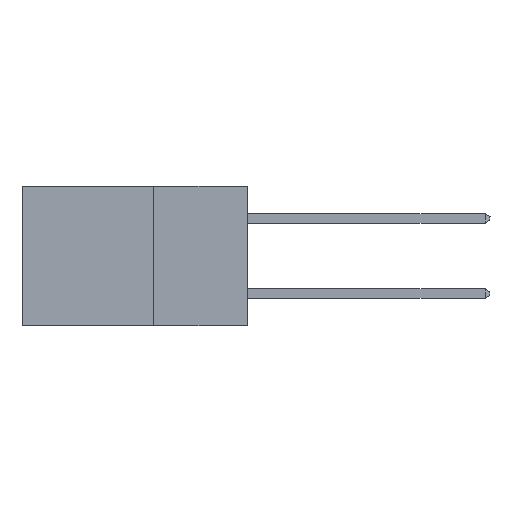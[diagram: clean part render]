
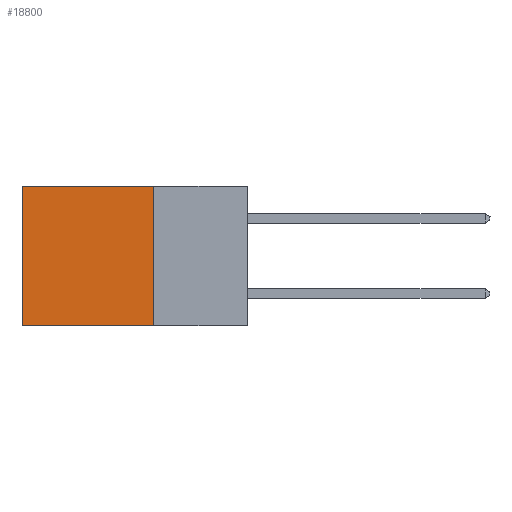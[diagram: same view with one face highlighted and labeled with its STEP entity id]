
A CAD part, left-side view. The second image highlights one B-rep face of the part: STEP entity #18800.
In plain terms, the highlighted planar face has unit normal (-1, 0, 0).
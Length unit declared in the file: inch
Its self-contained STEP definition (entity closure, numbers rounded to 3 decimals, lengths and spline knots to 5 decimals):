
#78 = CARTESIAN_POINT ( 'NONE',  ( 0.2615, 0.25, -0.37 ) ) ;
#239 = LINE ( 'NONE', #8650, #12060 ) ;
#1069 = ORIENTED_EDGE ( 'NONE', *, *, #21553, .F. ) ;
#3653 = VERTEX_POINT ( 'NONE', #22534 ) ;
#3857 = VECTOR ( 'NONE', #27031, 39.37008 ) ;
#5441 = LINE ( 'NONE', #24487, #11558 ) ;
#7405 = EDGE_CURVE ( 'NONE', #21974, #3653, #5441, .T. ) ;
#8078 = AXIS2_PLACEMENT_3D ( 'NONE', #11587, #19601, #15447 ) ;
#8094 = LINE ( 'NONE', #78, #11234 ) ;
#8464 = CARTESIAN_POINT ( 'NONE',  ( 0.2615, 0.25, -0.37 ) ) ;
#8650 = CARTESIAN_POINT ( 'NONE',  ( 0.2615, 0.6, -0.37 ) ) ;
#9124 = EDGE_CURVE ( 'NONE', #18058, #3653, #239, .T. ) ;
#9383 = ORIENTED_EDGE ( 'NONE', *, *, #10611, .T. ) ;
#10139 = CARTESIAN_POINT ( 'NONE',  ( 0.2615, 0.6, 0. ) ) ;
#10611 = EDGE_CURVE ( 'NONE', #21507, #18058, #21381, .T. ) ;
#11234 = VECTOR ( 'NONE', #19141, 39.37008 ) ;
#11558 = VECTOR ( 'NONE', #12071, 39.37008 ) ;
#11587 = CARTESIAN_POINT ( 'NONE',  ( 0.2615, 0.25, -0.37 ) ) ;
#12060 = VECTOR ( 'NONE', #17088, 39.37008 ) ;
#12071 = DIRECTION ( 'NONE',  ( 0., 1., 0. ) ) ;
#15447 = DIRECTION ( 'NONE',  ( 0., 0., -1. ) ) ;
#16134 = EDGE_LOOP ( 'NONE', ( #19415, #16583, #1069, #9383 ) ) ;
#16583 = ORIENTED_EDGE ( 'NONE', *, *, #7405, .F. ) ;
#17088 = DIRECTION ( 'NONE',  ( 0., 0., -1. ) ) ;
#17132 = CARTESIAN_POINT ( 'NONE',  ( 0.2615, 0.25, 0. ) ) ;
#18058 = VERTEX_POINT ( 'NONE', #10139 ) ;
#18800 = ADVANCED_FACE ( 'NONE', ( #22075 ), #22215, .F. ) ;
#18876 = CARTESIAN_POINT ( 'NONE',  ( 0.2615, 0.25, 0. ) ) ;
#19141 = DIRECTION ( 'NONE',  ( 0., 0., -1. ) ) ;
#19415 = ORIENTED_EDGE ( 'NONE', *, *, #9124, .T. ) ;
#19601 = DIRECTION ( 'NONE',  ( 1., 0., 0. ) ) ;
#21381 = LINE ( 'NONE', #17132, #3857 ) ;
#21507 = VERTEX_POINT ( 'NONE', #18876 ) ;
#21553 = EDGE_CURVE ( 'NONE', #21507, #21974, #8094, .T. ) ;
#21974 = VERTEX_POINT ( 'NONE', #8464 ) ;
#22075 = FACE_OUTER_BOUND ( 'NONE', #16134, .T. ) ;
#22215 = PLANE ( 'NONE',  #8078 ) ;
#22534 = CARTESIAN_POINT ( 'NONE',  ( 0.2615, 0.6, -0.37 ) ) ;
#24487 = CARTESIAN_POINT ( 'NONE',  ( 0.2615, 0.25, -0.37 ) ) ;
#27031 = DIRECTION ( 'NONE',  ( 0., 1., 0. ) ) ;
